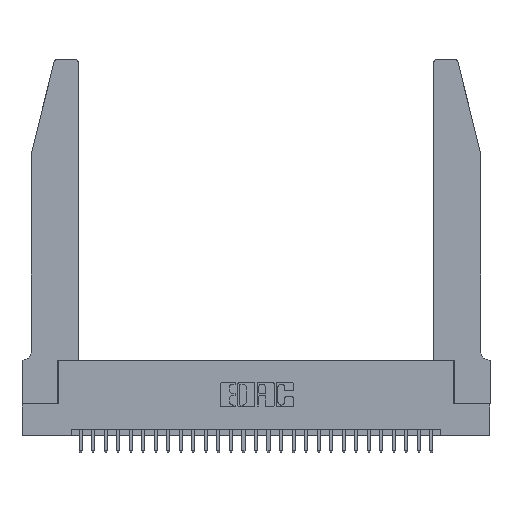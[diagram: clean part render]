
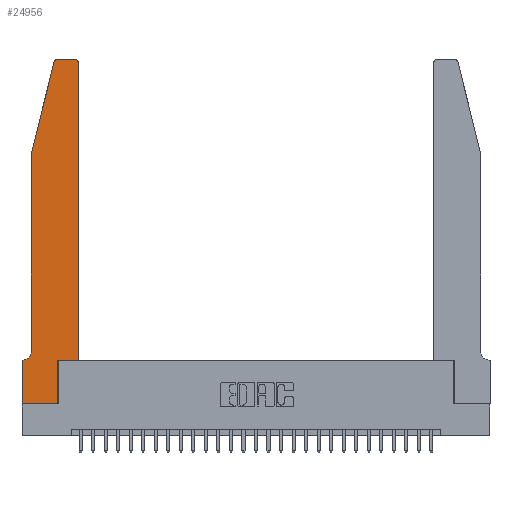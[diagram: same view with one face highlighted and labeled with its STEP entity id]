
A CAD part, top view. The second image highlights one B-rep face of the part: STEP entity #24956.
In plain terms, the highlighted planar face has unit normal (0, 0, 1).
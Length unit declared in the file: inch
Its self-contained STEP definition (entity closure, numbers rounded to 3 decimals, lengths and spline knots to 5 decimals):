
#79 = CIRCLE ( 'NONE', #385, 0.03 ) ;
#103 = LINE ( 'NONE', #4039, #22808 ) ;
#188 = VECTOR ( 'NONE', #9872, 39.37008 ) ;
#284 = CARTESIAN_POINT ( 'NONE',  ( 0.0755, 2., 0.37 ) ) ;
#385 = AXIS2_PLACEMENT_3D ( 'NONE', #28505, #15028, #1424 ) ;
#893 = ORIENTED_EDGE ( 'NONE', *, *, #8763, .T. ) ;
#1171 = VERTEX_POINT ( 'NONE', #4366 ) ;
#1424 = DIRECTION ( 'NONE',  ( 1., 0., 0. ) ) ;
#1831 = LINE ( 'NONE', #20213, #12470 ) ;
#2120 = DIRECTION ( 'NONE',  ( 0., 1., 0. ) ) ;
#2173 = EDGE_CURVE ( 'NONE', #24663, #25257, #11328, .T. ) ;
#2635 = ORIENTED_EDGE ( 'NONE', *, *, #11896, .T. ) ;
#2648 = DIRECTION ( 'NONE',  ( -0.239, -0.971, 0. ) ) ;
#2745 = VERTEX_POINT ( 'NONE', #19097 ) ;
#3163 = CARTESIAN_POINT ( 'NONE',  ( 0., 0., 0.37 ) ) ;
#3199 = EDGE_CURVE ( 'NONE', #11047, #25584, #27154, .T. ) ;
#3391 = CARTESIAN_POINT ( 'NONE',  ( 0.4505, 2.72, 0.37 ) ) ;
#3415 = FACE_OUTER_BOUND ( 'NONE', #4082, .T. ) ;
#4039 = CARTESIAN_POINT ( 'NONE',  ( 0.0755, 2., 0.37 ) ) ;
#4082 = EDGE_LOOP ( 'NONE', ( #20806, #6500, #893, #26193, #29187, #12102, #10369, #22980, #2635, #19415, #18776, #14175 ) ) ;
#4363 = CARTESIAN_POINT ( 'NONE',  ( 0., 0., 0.37 ) ) ;
#4366 = CARTESIAN_POINT ( 'NONE',  ( 0.2865, 0., 0.37 ) ) ;
#5807 = EDGE_CURVE ( 'NONE', #7623, #24498, #79, .T. ) ;
#6184 = AXIS2_PLACEMENT_3D ( 'NONE', #12075, #27935, #14459 ) ;
#6500 = ORIENTED_EDGE ( 'NONE', *, *, #22192, .T. ) ;
#6683 = DIRECTION ( 'NONE',  ( 1., 0., 0. ) ) ;
#7043 = EDGE_CURVE ( 'NONE', #2745, #11047, #24826, .T. ) ;
#7623 = VERTEX_POINT ( 'NONE', #3391 ) ;
#7628 = CARTESIAN_POINT ( 'NONE',  ( 0.4505, 0.35, 0.37 ) ) ;
#7676 = PLANE ( 'NONE',  #6184 ) ;
#8609 = AXIS2_PLACEMENT_3D ( 'NONE', #9989, #25755, #12240 ) ;
#8616 = DIRECTION ( 'NONE',  ( 0., -1., 0. ) ) ;
#8763 = EDGE_CURVE ( 'NONE', #10612, #21150, #22550, .T. ) ;
#8895 = EDGE_CURVE ( 'NONE', #25257, #7623, #18314, .T. ) ;
#9087 = DIRECTION ( 'NONE',  ( 0., 0., 1. ) ) ;
#9128 = VERTEX_POINT ( 'NONE', #10625 ) ;
#9872 = DIRECTION ( 'NONE',  ( 0., 1., 0. ) ) ;
#9989 = CARTESIAN_POINT ( 'NONE',  ( 0.0055, 0.42, 0.37 ) ) ;
#10034 = VERTEX_POINT ( 'NONE', #21065 ) ;
#10131 = CARTESIAN_POINT ( 'NONE',  ( 0., 0.35, 0.37 ) ) ;
#10350 = EDGE_CURVE ( 'NONE', #21150, #10034, #103, .T. ) ;
#10369 = ORIENTED_EDGE ( 'NONE', *, *, #3199, .T. ) ;
#10612 = VERTEX_POINT ( 'NONE', #17454 ) ;
#10615 = CARTESIAN_POINT ( 'NONE',  ( 0.0755, 0.35, 0.37 ) ) ;
#10625 = CARTESIAN_POINT ( 'NONE',  ( 0.284, 2.75, 0.37 ) ) ;
#11047 = VERTEX_POINT ( 'NONE', #10131 ) ;
#11328 = LINE ( 'NONE', #21778, #28599 ) ;
#11598 = EDGE_CURVE ( 'NONE', #10034, #2745, #14973, .T. ) ;
#11896 = EDGE_CURVE ( 'NONE', #1171, #24663, #1831, .T. ) ;
#12075 = CARTESIAN_POINT ( 'NONE',  ( 0., 0.35, 0.37 ) ) ;
#12102 = ORIENTED_EDGE ( 'NONE', *, *, #7043, .T. ) ;
#12240 = DIRECTION ( 'NONE',  ( -1., 0., 0. ) ) ;
#12340 = LINE ( 'NONE', #17596, #24361 ) ;
#12470 = VECTOR ( 'NONE', #2120, 39.37008 ) ;
#12799 = VECTOR ( 'NONE', #24147, 39.37008 ) ;
#13509 = CARTESIAN_POINT ( 'NONE',  ( 0.4505, 0.35, 0.37 ) ) ;
#14175 = ORIENTED_EDGE ( 'NONE', *, *, #5807, .T. ) ;
#14435 = DIRECTION ( 'NONE',  ( 0., -1., 0. ) ) ;
#14459 = DIRECTION ( 'NONE',  ( 1., 0., 0. ) ) ;
#14973 = CIRCLE ( 'NONE', #8609, 0.07 ) ;
#15028 = DIRECTION ( 'NONE',  ( 0., 0., 1. ) ) ;
#16319 = EDGE_CURVE ( 'NONE', #25584, #1171, #17643, .T. ) ;
#17454 = CARTESIAN_POINT ( 'NONE',  ( 0.25487, 2.72718, 0.37 ) ) ;
#17596 = CARTESIAN_POINT ( 'NONE',  ( 0.2605, 2.75, 0.37 ) ) ;
#17643 = LINE ( 'NONE', #4363, #18356 ) ;
#18314 = LINE ( 'NONE', #7628, #188 ) ;
#18356 = VECTOR ( 'NONE', #6683, 39.37008 ) ;
#18776 = ORIENTED_EDGE ( 'NONE', *, *, #8895, .T. ) ;
#18791 = CIRCLE ( 'NONE', #21826, 0.03 ) ;
#19097 = CARTESIAN_POINT ( 'NONE',  ( 0.0055, 0.35, 0.37 ) ) ;
#19415 = ORIENTED_EDGE ( 'NONE', *, *, #2173, .T. ) ;
#19603 = CARTESIAN_POINT ( 'NONE',  ( 0.4205, 2.75, 0.37 ) ) ;
#19851 = DIRECTION ( 'NONE',  ( -1., 0., 0. ) ) ;
#20213 = CARTESIAN_POINT ( 'NONE',  ( 0.2865, 0.35, 0.37 ) ) ;
#20806 = ORIENTED_EDGE ( 'NONE', *, *, #23395, .T. ) ;
#21065 = CARTESIAN_POINT ( 'NONE',  ( 0.0755, 0.42, 0.37 ) ) ;
#21150 = VERTEX_POINT ( 'NONE', #22097 ) ;
#21176 = VECTOR ( 'NONE', #14435, 39.37008 ) ;
#21778 = CARTESIAN_POINT ( 'NONE',  ( 0.4505, 0.35, 0.37 ) ) ;
#21826 = AXIS2_PLACEMENT_3D ( 'NONE', #22578, #9087, #24856 ) ;
#21851 = VECTOR ( 'NONE', #2648, 39.37008 ) ;
#22097 = CARTESIAN_POINT ( 'NONE',  ( 0.0755, 2., 0.37 ) ) ;
#22192 = EDGE_CURVE ( 'NONE', #9128, #10612, #18791, .T. ) ;
#22550 = LINE ( 'NONE', #284, #21851 ) ;
#22578 = CARTESIAN_POINT ( 'NONE',  ( 0.284, 2.72, 0.37 ) ) ;
#22808 = VECTOR ( 'NONE', #8616, 39.37008 ) ;
#22980 = ORIENTED_EDGE ( 'NONE', *, *, #16319, .T. ) ;
#23395 = EDGE_CURVE ( 'NONE', #24498, #9128, #12340, .T. ) ;
#24057 = DIRECTION ( 'NONE',  ( 1., 0., 0. ) ) ;
#24147 = DIRECTION ( 'NONE',  ( -1., 0., 0. ) ) ;
#24361 = VECTOR ( 'NONE', #19851, 39.37008 ) ;
#24498 = VERTEX_POINT ( 'NONE', #19603 ) ;
#24663 = VERTEX_POINT ( 'NONE', #29205 ) ;
#24826 = LINE ( 'NONE', #10615, #12799 ) ;
#24856 = DIRECTION ( 'NONE',  ( 1., 0., 0. ) ) ;
#24956 = ADVANCED_FACE ( 'NONE', ( #3415 ), #7676, .T. ) ;
#25257 = VERTEX_POINT ( 'NONE', #13509 ) ;
#25584 = VERTEX_POINT ( 'NONE', #25748 ) ;
#25748 = CARTESIAN_POINT ( 'NONE',  ( 0., 0., 0.37 ) ) ;
#25755 = DIRECTION ( 'NONE',  ( 0., 0., -1. ) ) ;
#26193 = ORIENTED_EDGE ( 'NONE', *, *, #10350, .T. ) ;
#27154 = LINE ( 'NONE', #3163, #21176 ) ;
#27935 = DIRECTION ( 'NONE',  ( 0., 0., 1. ) ) ;
#28505 = CARTESIAN_POINT ( 'NONE',  ( 0.4205, 2.72, 0.37 ) ) ;
#28599 = VECTOR ( 'NONE', #24057, 39.37008 ) ;
#29187 = ORIENTED_EDGE ( 'NONE', *, *, #11598, .T. ) ;
#29205 = CARTESIAN_POINT ( 'NONE',  ( 0.2865, 0.35, 0.37 ) ) ;
